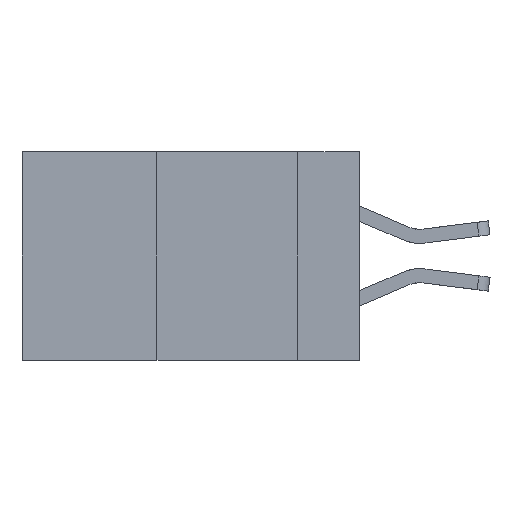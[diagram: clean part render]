
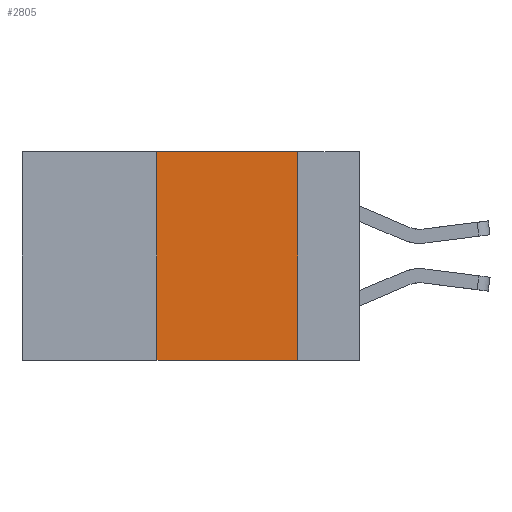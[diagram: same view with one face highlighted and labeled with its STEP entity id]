
A CAD part, left-side view. The second image highlights one B-rep face of the part: STEP entity #2805.
In plain terms, the highlighted planar face has unit normal (-1, 0, 0).
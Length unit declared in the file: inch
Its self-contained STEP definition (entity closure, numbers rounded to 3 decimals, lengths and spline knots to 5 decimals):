
#111 = CARTESIAN_POINT ( 'NONE',  ( 0., 0.36, -0.37 ) ) ;
#162 = DIRECTION ( 'NONE',  ( 0., -1., 0. ) ) ;
#196 = DIRECTION ( 'NONE',  ( 0., 0., -1. ) ) ;
#262 = VECTOR ( 'NONE', #7521, 39.37008 ) ;
#468 = VECTOR ( 'NONE', #196, 39.37008 ) ;
#1059 = VECTOR ( 'NONE', #162, 39.37008 ) ;
#1658 = CARTESIAN_POINT ( 'NONE',  ( 0., 0.11, 0. ) ) ;
#1668 = EDGE_CURVE ( 'NONE', #2566, #8914, #7994, .T. ) ;
#2566 = VERTEX_POINT ( 'NONE', #111 ) ;
#2610 = PLANE ( 'NONE',  #14550 ) ;
#2805 = ADVANCED_FACE ( 'NONE', ( #12180 ), #2610, .F. ) ;
#3174 = ORIENTED_EDGE ( 'NONE', *, *, #7434, .T. ) ;
#3348 = VERTEX_POINT ( 'NONE', #13249 ) ;
#3769 = DIRECTION ( 'NONE',  ( 0., 0., -1. ) ) ;
#3796 = VERTEX_POINT ( 'NONE', #1658 ) ;
#4512 = LINE ( 'NONE', #9433, #1059 ) ;
#5135 = EDGE_LOOP ( 'NONE', ( #12175, #12846, #9233, #3174 ) ) ;
#6311 = DIRECTION ( 'NONE',  ( 1., 0., 0. ) ) ;
#7178 = CARTESIAN_POINT ( 'NONE',  ( 0., 0.11, 0. ) ) ;
#7434 = EDGE_CURVE ( 'NONE', #2566, #3348, #4512, .T. ) ;
#7521 = DIRECTION ( 'NONE',  ( 0., -1., 0. ) ) ;
#7994 = LINE ( 'NONE', #10756, #13184 ) ;
#8914 = VERTEX_POINT ( 'NONE', #13100 ) ;
#9233 = ORIENTED_EDGE ( 'NONE', *, *, #1668, .F. ) ;
#9433 = CARTESIAN_POINT ( 'NONE',  ( 0., 0.6, -0.37 ) ) ;
#9485 = LINE ( 'NONE', #14040, #262 ) ;
#10745 = CARTESIAN_POINT ( 'NONE',  ( 0., 0.6, 0. ) ) ;
#10756 = CARTESIAN_POINT ( 'NONE',  ( 0., 0.36, 0. ) ) ;
#11962 = DIRECTION ( 'NONE',  ( 0., 0., 1. ) ) ;
#12175 = ORIENTED_EDGE ( 'NONE', *, *, #12663, .F. ) ;
#12180 = FACE_OUTER_BOUND ( 'NONE', #5135, .T. ) ;
#12278 = LINE ( 'NONE', #7178, #468 ) ;
#12663 = EDGE_CURVE ( 'NONE', #3796, #3348, #12278, .T. ) ;
#12846 = ORIENTED_EDGE ( 'NONE', *, *, #12900, .F. ) ;
#12900 = EDGE_CURVE ( 'NONE', #8914, #3796, #9485, .T. ) ;
#13100 = CARTESIAN_POINT ( 'NONE',  ( 0., 0.36, 0. ) ) ;
#13184 = VECTOR ( 'NONE', #11962, 39.37008 ) ;
#13249 = CARTESIAN_POINT ( 'NONE',  ( 0., 0.11, -0.37 ) ) ;
#14040 = CARTESIAN_POINT ( 'NONE',  ( 0., 0.6, 0. ) ) ;
#14550 = AXIS2_PLACEMENT_3D ( 'NONE', #10745, #6311, #3769 ) ;
